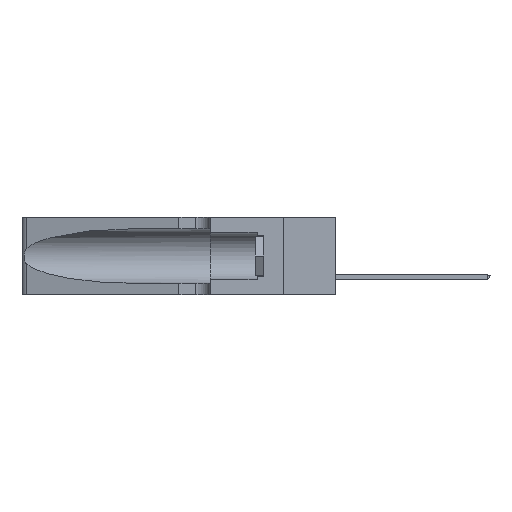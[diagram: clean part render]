
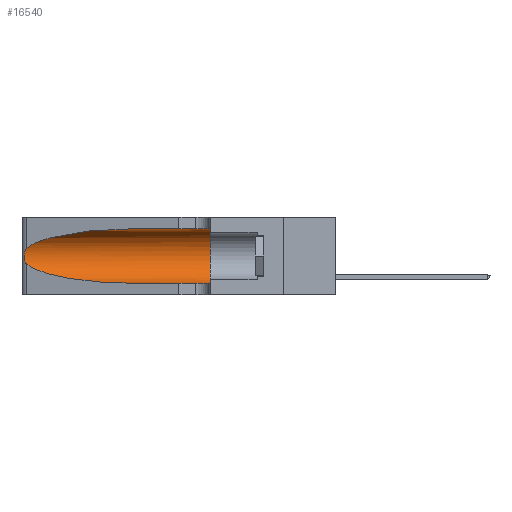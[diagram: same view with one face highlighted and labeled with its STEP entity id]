
A CAD part, left-side view. The second image highlights one B-rep face of the part: STEP entity #16540.
In plain terms, the highlighted cylindrical face has radius 3.308 mm (diameter 6.617 mm), a partial arc.
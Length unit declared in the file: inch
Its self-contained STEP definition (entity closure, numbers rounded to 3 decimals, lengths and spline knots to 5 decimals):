
#376 = ORIENTED_EDGE ( 'NONE', *, *, #23891, .T. ) ;
#723 = AXIS2_PLACEMENT_3D ( 'NONE', #12065, #28332, #21751 ) ;
#1536 = ORIENTED_EDGE ( 'NONE', *, *, #27881, .T. ) ;
#1586 =( BOUNDED_CURVE ( )  B_SPLINE_CURVE ( 3, ( #22288, #3103, #5479, #5684 ),
 .UNSPECIFIED., .F., .T. ) 
 B_SPLINE_CURVE_WITH_KNOTS ( ( 4, 4 ),
 ( 1.5708, 2.84003 ),
 .UNSPECIFIED. ) 
 CURVE ( )  GEOMETRIC_REPRESENTATION_ITEM ( )  RATIONAL_B_SPLINE_CURVE ( ( 1., 0.87, 0.87, 1. ) ) 
 REPRESENTATION_ITEM ( '' )  );
#2345 = EDGE_CURVE ( 'NONE', #19142, #20518, #1586, .T. ) ;
#2766 = EDGE_CURVE ( 'NONE', #21862, #29249, #22266, .T. ) ;
#3103 = CARTESIAN_POINT ( 'NONE',  ( 0.18966, 0.96281, 0.31525 ) ) ;
#3186 = CARTESIAN_POINT ( 'NONE',  ( 0.1305, 0.35, 0.185 ) ) ;
#4188 = CARTESIAN_POINT ( 'NONE',  ( 0.26075, 1.23896, 0.19203 ) ) ;
#4489 = CARTESIAN_POINT ( 'NONE',  ( 0.26017, 1.23833, 0.17102 ) ) ;
#5100 = CARTESIAN_POINT ( 'NONE',  ( 0.25487, 1.22718, 0.14631 ) ) ;
#5479 = CARTESIAN_POINT ( 'NONE',  ( 0.2373, 1.15595, 0.28018 ) ) ;
#5684 = CARTESIAN_POINT ( 'NONE',  ( 0.25487, 1.22718, 0.22369 ) ) ;
#6379 = CARTESIAN_POINT ( 'NONE',  ( 0.1305, 0.35, 0.31525 ) ) ;
#6542 = CARTESIAN_POINT ( 'NONE',  ( 0.26075, 1.23896, 0.178 ) ) ;
#7415 = CARTESIAN_POINT ( 'NONE',  ( 0.1305, 1.61858, 0.05475 ) ) ;
#7517 = DIRECTION ( 'NONE',  ( 0., -1., 0. ) ) ;
#7675 = CARTESIAN_POINT ( 'NONE',  ( 0.2373, 1.15595, 0.08982 ) ) ;
#7907 = CARTESIAN_POINT ( 'NONE',  ( 0.25487, 1.22718, 0.22369 ) ) ;
#8551 = CARTESIAN_POINT ( 'NONE',  ( 0.1305, 1.61858, 0.31525 ) ) ;
#8932 = CARTESIAN_POINT ( 'NONE',  ( 0.25787, 1.23484, 0.2124 ) ) ;
#9023 = LINE ( 'NONE', #8551, #14123 ) ;
#9221 = ORIENTED_EDGE ( 'NONE', *, *, #18227, .F. ) ;
#9387 = CARTESIAN_POINT ( 'NONE',  ( 0.1305, 0.72297, 0.31525 ) ) ;
#10072 = CARTESIAN_POINT ( 'NONE',  ( 0.18966, 0.96281, 0.05475 ) ) ;
#10499 = DIRECTION ( 'NONE',  ( 0., 0., 1. ) ) ;
#10974 = CARTESIAN_POINT ( 'NONE',  ( 0.25487, 1.22718, 0.22369 ) ) ;
#11171 = AXIS2_PLACEMENT_3D ( 'NONE', #3186, #19993, #10499 ) ;
#11593 = CARTESIAN_POINT ( 'NONE',  ( 0.25555, 1.22993, 0.14849 ) ) ;
#12065 = CARTESIAN_POINT ( 'NONE',  ( 0.1305, 1.61858, 0.185 ) ) ;
#12203 = LINE ( 'NONE', #7415, #21780 ) ;
#12293 = EDGE_LOOP ( 'NONE', ( #23352, #376, #1536, #27465, #26035, #9221 ) ) ;
#13559 = CARTESIAN_POINT ( 'NONE',  ( 0.26018, 1.23835, 0.19895 ) ) ;
#14039 = CARTESIAN_POINT ( 'NONE',  ( 0.25487, 1.22718, 0.14631 ) ) ;
#14123 = VECTOR ( 'NONE', #25058, 39.37008 ) ;
#15198 = B_SPLINE_CURVE_WITH_KNOTS ( 'NONE', 3,
 ( #10974, #15752, #18319, #8932, #25306, #13559, #4188, #6542, #4489, #20972, #18915, #28139, #11593, #14039 ),
 .UNSPECIFIED., .F., .F.,
 ( 4, 2, 2, 2, 2, 2, 4 ),
 ( 0., 0.00027, 0.00053, 0.00107, 0.0016, 0.00187, 0.00214 ),
 .UNSPECIFIED. ) ;
#15752 = CARTESIAN_POINT ( 'NONE',  ( 0.25555, 1.22994, 0.2215 ) ) ;
#16540 = ADVANCED_FACE ( 'NONE', ( #29315 ), #28209, .F. ) ;
#16857 = CARTESIAN_POINT ( 'NONE',  ( 0.1305, 0.72297, 0.05475 ) ) ;
#18227 = EDGE_CURVE ( 'NONE', #19142, #21862, #9023, .T. ) ;
#18319 = CARTESIAN_POINT ( 'NONE',  ( 0.25639, 1.23184, 0.21858 ) ) ;
#18321 = CARTESIAN_POINT ( 'NONE',  ( 0.1305, 0.35, 0.05475 ) ) ;
#18915 = CARTESIAN_POINT ( 'NONE',  ( 0.25789, 1.23486, 0.15765 ) ) ;
#19142 = VERTEX_POINT ( 'NONE', #9387 ) ;
#19942 =( BOUNDED_CURVE ( )  B_SPLINE_CURVE ( 3, ( #5100, #7675, #10072, #26341 ),
 .UNSPECIFIED., .F., .T. ) 
 B_SPLINE_CURVE_WITH_KNOTS ( ( 4, 4 ),
 ( 3.44316, 4.71239 ),
 .UNSPECIFIED. ) 
 CURVE ( )  GEOMETRIC_REPRESENTATION_ITEM ( )  RATIONAL_B_SPLINE_CURVE ( ( 1., 0.87, 0.87, 1. ) ) 
 REPRESENTATION_ITEM ( '' )  );
#19993 = DIRECTION ( 'NONE',  ( 0., 1., 0. ) ) ;
#20518 = VERTEX_POINT ( 'NONE', #7907 ) ;
#20972 = CARTESIAN_POINT ( 'NONE',  ( 0.25856, 1.23593, 0.16098 ) ) ;
#21751 = DIRECTION ( 'NONE',  ( 0., 0., -1. ) ) ;
#21780 = VECTOR ( 'NONE', #7517, 39.37008 ) ;
#21862 = VERTEX_POINT ( 'NONE', #6379 ) ;
#22266 = CIRCLE ( 'NONE', #11171, 0.13025 ) ;
#22288 = CARTESIAN_POINT ( 'NONE',  ( 0.1305, 0.72297, 0.31525 ) ) ;
#23352 = ORIENTED_EDGE ( 'NONE', *, *, #2345, .T. ) ;
#23759 = EDGE_CURVE ( 'NONE', #27267, #29249, #12203, .T. ) ;
#23891 = EDGE_CURVE ( 'NONE', #20518, #24720, #15198, .T. ) ;
#24720 = VERTEX_POINT ( 'NONE', #28503 ) ;
#25058 = DIRECTION ( 'NONE',  ( 0., -1., 0. ) ) ;
#25306 = CARTESIAN_POINT ( 'NONE',  ( 0.25854, 1.2359, 0.20912 ) ) ;
#26035 = ORIENTED_EDGE ( 'NONE', *, *, #2766, .F. ) ;
#26341 = CARTESIAN_POINT ( 'NONE',  ( 0.1305, 0.72297, 0.05475 ) ) ;
#27267 = VERTEX_POINT ( 'NONE', #16857 ) ;
#27465 = ORIENTED_EDGE ( 'NONE', *, *, #23759, .T. ) ;
#27881 = EDGE_CURVE ( 'NONE', #24720, #27267, #19942, .T. ) ;
#28139 = CARTESIAN_POINT ( 'NONE',  ( 0.25639, 1.23186, 0.15144 ) ) ;
#28209 = CYLINDRICAL_SURFACE ( 'NONE', #723, 0.13025 ) ;
#28332 = DIRECTION ( 'NONE',  ( 0., -1., 0. ) ) ;
#28503 = CARTESIAN_POINT ( 'NONE',  ( 0.25487, 1.22718, 0.14631 ) ) ;
#29249 = VERTEX_POINT ( 'NONE', #18321 ) ;
#29315 = FACE_OUTER_BOUND ( 'NONE', #12293, .T. ) ;
